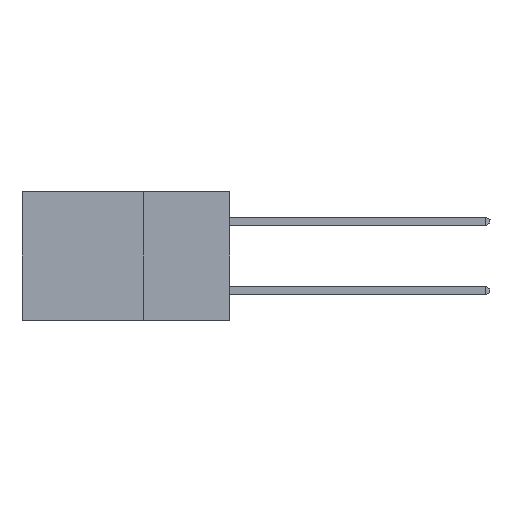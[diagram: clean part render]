
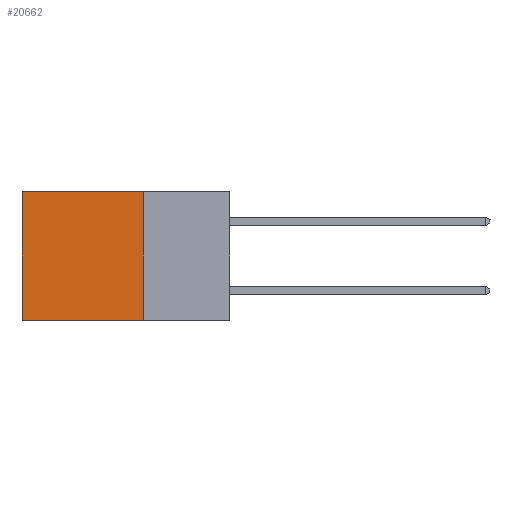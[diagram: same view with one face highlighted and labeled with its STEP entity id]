
A CAD part, left-side view. The second image highlights one B-rep face of the part: STEP entity #20662.
In plain terms, the highlighted planar face has unit normal (-1, 0, 0).
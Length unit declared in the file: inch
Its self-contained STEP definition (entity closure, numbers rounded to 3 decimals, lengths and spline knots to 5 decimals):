
#268 = ORIENTED_EDGE ( 'NONE', *, *, #14920, .F. ) ;
#543 = DIRECTION ( 'NONE',  ( 0., 0., -1. ) ) ;
#727 = VECTOR ( 'NONE', #6325, 39.37008 ) ;
#910 = CARTESIAN_POINT ( 'NONE',  ( 0.298, 0.6, -0.37 ) ) ;
#1384 = EDGE_LOOP ( 'NONE', ( #5715, #25451, #268, #3095 ) ) ;
#3069 = LINE ( 'NONE', #3617, #13222 ) ;
#3095 = ORIENTED_EDGE ( 'NONE', *, *, #13304, .T. ) ;
#3252 = AXIS2_PLACEMENT_3D ( 'NONE', #4377, #8348, #21593 ) ;
#3550 = LINE ( 'NONE', #15014, #13740 ) ;
#3617 = CARTESIAN_POINT ( 'NONE',  ( 0.298, 0.6, 0. ) ) ;
#3859 = LINE ( 'NONE', #21978, #11634 ) ;
#4185 = DIRECTION ( 'NONE',  ( 0., 1., 0. ) ) ;
#4248 = VERTEX_POINT ( 'NONE', #13570 ) ;
#4377 = CARTESIAN_POINT ( 'NONE',  ( 0.298, 0.25, 0. ) ) ;
#5666 = CARTESIAN_POINT ( 'NONE',  ( 0.298, 0.25, -0.37 ) ) ;
#5715 = ORIENTED_EDGE ( 'NONE', *, *, #17116, .T. ) ;
#6325 = DIRECTION ( 'NONE',  ( 0., 1., 0. ) ) ;
#8348 = DIRECTION ( 'NONE',  ( 1., 0., 0. ) ) ;
#8827 = CARTESIAN_POINT ( 'NONE',  ( 0.298, 0.25, 0. ) ) ;
#8970 = VERTEX_POINT ( 'NONE', #910 ) ;
#10296 = EDGE_CURVE ( 'NONE', #4248, #8970, #26721, .T. ) ;
#11634 = VECTOR ( 'NONE', #543, 39.37008 ) ;
#13222 = VECTOR ( 'NONE', #18780, 39.37008 ) ;
#13304 = EDGE_CURVE ( 'NONE', #15604, #23043, #3550, .T. ) ;
#13570 = CARTESIAN_POINT ( 'NONE',  ( 0.298, 0.25, -0.37 ) ) ;
#13740 = VECTOR ( 'NONE', #4185, 39.37008 ) ;
#14920 = EDGE_CURVE ( 'NONE', #15604, #4248, #3859, .T. ) ;
#15013 = PLANE ( 'NONE',  #3252 ) ;
#15014 = CARTESIAN_POINT ( 'NONE',  ( 0.298, 0.25, 0. ) ) ;
#15604 = VERTEX_POINT ( 'NONE', #8827 ) ;
#17116 = EDGE_CURVE ( 'NONE', #23043, #8970, #3069, .T. ) ;
#18780 = DIRECTION ( 'NONE',  ( 0., 0., -1. ) ) ;
#20662 = ADVANCED_FACE ( 'NONE', ( #21831 ), #15013, .F. ) ;
#21593 = DIRECTION ( 'NONE',  ( 0., 0., -1. ) ) ;
#21831 = FACE_OUTER_BOUND ( 'NONE', #1384, .T. ) ;
#21978 = CARTESIAN_POINT ( 'NONE',  ( 0.298, 0.25, 0. ) ) ;
#22042 = CARTESIAN_POINT ( 'NONE',  ( 0.298, 0.6, 0. ) ) ;
#23043 = VERTEX_POINT ( 'NONE', #22042 ) ;
#25451 = ORIENTED_EDGE ( 'NONE', *, *, #10296, .F. ) ;
#26721 = LINE ( 'NONE', #5666, #727 ) ;
